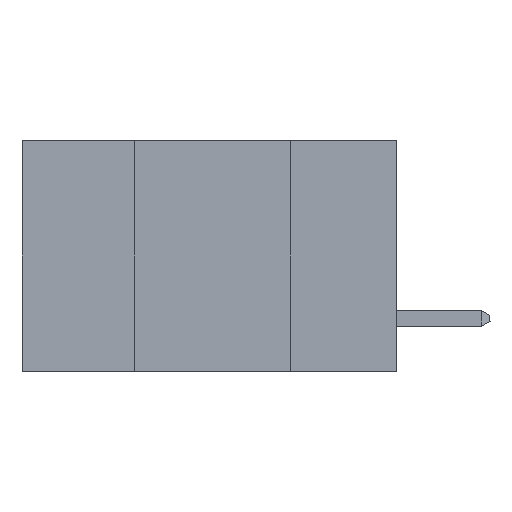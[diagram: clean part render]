
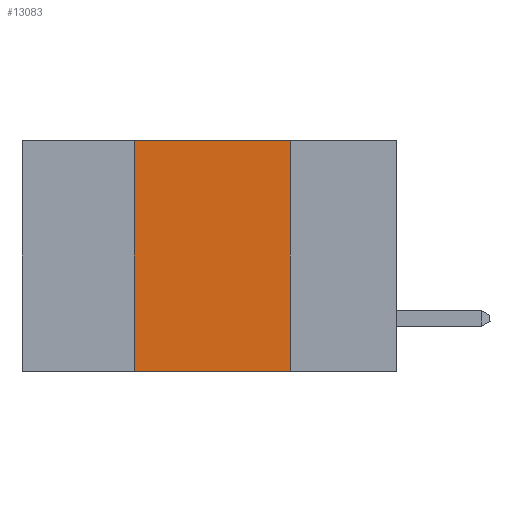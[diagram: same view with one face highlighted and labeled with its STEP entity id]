
A CAD part, left-side view. The second image highlights one B-rep face of the part: STEP entity #13083.
In plain terms, the highlighted planar face has unit normal (-1, 0, 0).
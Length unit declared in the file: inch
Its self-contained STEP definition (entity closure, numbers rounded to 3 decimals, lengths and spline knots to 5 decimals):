
#2057 = EDGE_CURVE ( 'NONE', #5697, #2241, #14735, .T. ) ;
#2241 = VERTEX_POINT ( 'NONE', #3212 ) ;
#2543 = VECTOR ( 'NONE', #13909, 39.37008 ) ;
#2840 = DIRECTION ( 'NONE',  ( 0., 0., 1. ) ) ;
#3185 = EDGE_CURVE ( 'NONE', #5036, #3191, #13795, .T. ) ;
#3191 = VERTEX_POINT ( 'NONE', #11082 ) ;
#3212 = CARTESIAN_POINT ( 'NONE',  ( 0., 0.17, -0.37 ) ) ;
#3592 = CARTESIAN_POINT ( 'NONE',  ( 0., 0.17, 0. ) ) ;
#4217 = DIRECTION ( 'NONE',  ( 0., -1., 0. ) ) ;
#4556 = PLANE ( 'NONE',  #8479 ) ;
#5036 = VERTEX_POINT ( 'NONE', #6194 ) ;
#5697 = VERTEX_POINT ( 'NONE', #3592 ) ;
#5766 = CARTESIAN_POINT ( 'NONE',  ( 0., 0.6, 0. ) ) ;
#5817 = DIRECTION ( 'NONE',  ( 0., 0., -1. ) ) ;
#5868 = EDGE_CURVE ( 'NONE', #5036, #2241, #12795, .T. ) ;
#6194 = CARTESIAN_POINT ( 'NONE',  ( 0., 0.42, -0.37 ) ) ;
#6262 = ORIENTED_EDGE ( 'NONE', *, *, #12052, .F. ) ;
#6465 = VECTOR ( 'NONE', #8637, 39.37008 ) ;
#6832 = ORIENTED_EDGE ( 'NONE', *, *, #5868, .T. ) ;
#6835 = LINE ( 'NONE', #12078, #6465 ) ;
#6989 = EDGE_LOOP ( 'NONE', ( #12249, #6262, #14774, #6832 ) ) ;
#7892 = CARTESIAN_POINT ( 'NONE',  ( 0., 0.6, -0.37 ) ) ;
#8479 = AXIS2_PLACEMENT_3D ( 'NONE', #5766, #12785, #5817 ) ;
#8637 = DIRECTION ( 'NONE',  ( 0., -1., 0. ) ) ;
#9365 = FACE_OUTER_BOUND ( 'NONE', #6989, .T. ) ;
#9384 = VECTOR ( 'NONE', #4217, 39.37008 ) ;
#10406 = VECTOR ( 'NONE', #2840, 39.37008 ) ;
#11082 = CARTESIAN_POINT ( 'NONE',  ( 0., 0.42, 0. ) ) ;
#12052 = EDGE_CURVE ( 'NONE', #3191, #5697, #6835, .T. ) ;
#12078 = CARTESIAN_POINT ( 'NONE',  ( 0., 0.6, 0. ) ) ;
#12247 = CARTESIAN_POINT ( 'NONE',  ( 0., 0.42, 0. ) ) ;
#12249 = ORIENTED_EDGE ( 'NONE', *, *, #2057, .F. ) ;
#12785 = DIRECTION ( 'NONE',  ( 1., 0., 0. ) ) ;
#12795 = LINE ( 'NONE', #7892, #9384 ) ;
#13083 = ADVANCED_FACE ( 'NONE', ( #9365 ), #4556, .F. ) ;
#13795 = LINE ( 'NONE', #12247, #10406 ) ;
#13909 = DIRECTION ( 'NONE',  ( 0., 0., -1. ) ) ;
#14707 = CARTESIAN_POINT ( 'NONE',  ( 0., 0.17, 0. ) ) ;
#14735 = LINE ( 'NONE', #14707, #2543 ) ;
#14774 = ORIENTED_EDGE ( 'NONE', *, *, #3185, .F. ) ;
